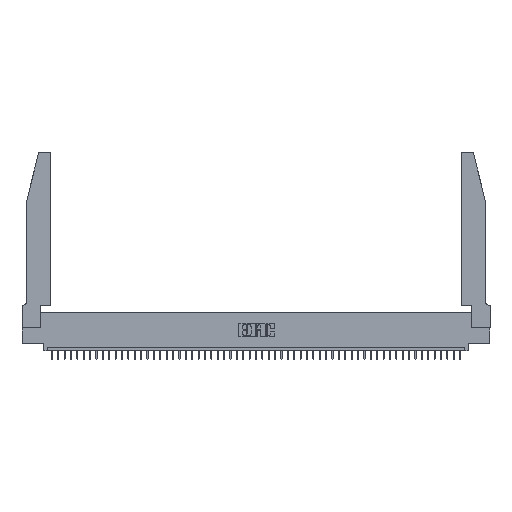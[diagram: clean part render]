
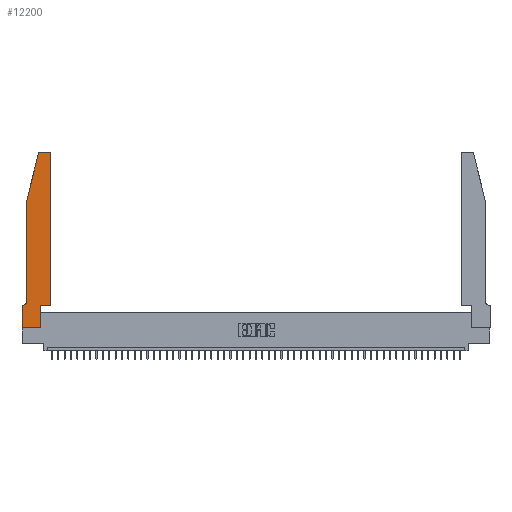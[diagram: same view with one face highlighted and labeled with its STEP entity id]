
A CAD part, top view. The second image highlights one B-rep face of the part: STEP entity #12200.
In plain terms, the highlighted planar face has unit normal (0, 0, 1).
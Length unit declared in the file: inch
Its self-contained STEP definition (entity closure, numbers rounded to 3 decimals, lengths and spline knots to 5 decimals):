
#58 = EDGE_CURVE ( 'NONE', #9470, #3059, #21511, .T. ) ;
#672 = VERTEX_POINT ( 'NONE', #29028 ) ;
#1296 = CARTESIAN_POINT ( 'NONE',  ( 0., 0., 0.37 ) ) ;
#1304 = DIRECTION ( 'NONE',  ( 0., -1., 0. ) ) ;
#2392 = LINE ( 'NONE', #41410, #19967 ) ;
#2555 = EDGE_CURVE ( 'NONE', #45076, #46484, #17953, .T. ) ;
#2768 = AXIS2_PLACEMENT_3D ( 'NONE', #23209, #31160, #35787 ) ;
#2921 = CARTESIAN_POINT ( 'NONE',  ( 0.4505, 2.72, 0.37 ) ) ;
#3059 = VERTEX_POINT ( 'NONE', #1296 ) ;
#3285 = CARTESIAN_POINT ( 'NONE',  ( 0.4205, 2.72, 0.37 ) ) ;
#4116 = EDGE_CURVE ( 'NONE', #12988, #48540, #21064, .T. ) ;
#4312 = DIRECTION ( 'NONE',  ( 0., 0., -1. ) ) ;
#4430 = CARTESIAN_POINT ( 'NONE',  ( 0.0755, 0.35, 0.37 ) ) ;
#5027 = ORIENTED_EDGE ( 'NONE', *, *, #22944, .T. ) ;
#6614 = VECTOR ( 'NONE', #42459, 39.37008 ) ;
#7496 = LINE ( 'NONE', #4430, #47885 ) ;
#7932 = CARTESIAN_POINT ( 'NONE',  ( 0.284, 2.72, 0.37 ) ) ;
#8965 = VERTEX_POINT ( 'NONE', #11845 ) ;
#9470 = VERTEX_POINT ( 'NONE', #25887 ) ;
#9609 = LINE ( 'NONE', #37846, #50065 ) ;
#9868 = ORIENTED_EDGE ( 'NONE', *, *, #12426, .T. ) ;
#9966 = EDGE_CURVE ( 'NONE', #14212, #9470, #7496, .T. ) ;
#10384 = DIRECTION ( 'NONE',  ( 1., 0., 0. ) ) ;
#10969 = DIRECTION ( 'NONE',  ( 0., 0., 1. ) ) ;
#11072 = CIRCLE ( 'NONE', #14379, 0.03 ) ;
#11243 = AXIS2_PLACEMENT_3D ( 'NONE', #20483, #4312, #31771 ) ;
#11390 = PLANE ( 'NONE',  #2768 ) ;
#11602 = DIRECTION ( 'NONE',  ( -1., 0., 0. ) ) ;
#11845 = CARTESIAN_POINT ( 'NONE',  ( 0.284, 2.75, 0.37 ) ) ;
#12200 = ADVANCED_FACE ( 'NONE', ( #46612 ), #11390, .T. ) ;
#12426 = EDGE_CURVE ( 'NONE', #46484, #8965, #2392, .T. ) ;
#12988 = VERTEX_POINT ( 'NONE', #14628 ) ;
#13053 = AXIS2_PLACEMENT_3D ( 'NONE', #3285, #10969, #22793 ) ;
#13166 = ORIENTED_EDGE ( 'NONE', *, *, #58, .T. ) ;
#13350 = DIRECTION ( 'NONE',  ( -0.239, -0.971, 0. ) ) ;
#13462 = ORIENTED_EDGE ( 'NONE', *, *, #22969, .T. ) ;
#13710 = DIRECTION ( 'NONE',  ( 0., 1., 0. ) ) ;
#13948 = VECTOR ( 'NONE', #13710, 39.37008 ) ;
#14212 = VERTEX_POINT ( 'NONE', #38757 ) ;
#14379 = AXIS2_PLACEMENT_3D ( 'NONE', #7932, #32320, #24113 ) ;
#14628 = CARTESIAN_POINT ( 'NONE',  ( 0.0755, 2., 0.37 ) ) ;
#14653 = VERTEX_POINT ( 'NONE', #38193 ) ;
#16464 = VECTOR ( 'NONE', #10384, 39.37008 ) ;
#16563 = EDGE_CURVE ( 'NONE', #48540, #14212, #21930, .T. ) ;
#17202 = CARTESIAN_POINT ( 'NONE',  ( 0.0755, 2., 0.37 ) ) ;
#17310 = CARTESIAN_POINT ( 'NONE',  ( 0.4505, 0.35, 0.37 ) ) ;
#17953 = CIRCLE ( 'NONE', #13053, 0.03 ) ;
#17994 = CARTESIAN_POINT ( 'NONE',  ( 0.4205, 2.75, 0.37 ) ) ;
#19967 = VECTOR ( 'NONE', #41155, 39.37008 ) ;
#20011 = ORIENTED_EDGE ( 'NONE', *, *, #30833, .T. ) ;
#20483 = CARTESIAN_POINT ( 'NONE',  ( 0.0055, 0.42, 0.37 ) ) ;
#21064 = LINE ( 'NONE', #25414, #48483 ) ;
#21511 = LINE ( 'NONE', #37184, #28459 ) ;
#21930 = CIRCLE ( 'NONE', #11243, 0.07 ) ;
#22286 = ORIENTED_EDGE ( 'NONE', *, *, #2555, .T. ) ;
#22441 = LINE ( 'NONE', #33747, #16464 ) ;
#22793 = DIRECTION ( 'NONE',  ( 1., 0., 0. ) ) ;
#22944 = EDGE_CURVE ( 'NONE', #14653, #45076, #36853, .T. ) ;
#22969 = EDGE_CURVE ( 'NONE', #28114, #672, #9609, .T. ) ;
#23209 = CARTESIAN_POINT ( 'NONE',  ( 0., 0.35, 0.37 ) ) ;
#24113 = DIRECTION ( 'NONE',  ( 1., 0., 0. ) ) ;
#24419 = EDGE_CURVE ( 'NONE', #3059, #28114, #27297, .T. ) ;
#24710 = EDGE_LOOP ( 'NONE', ( #9868, #20011, #31247, #25897, #38358, #29701, #13166, #38920, #13462, #40900, #5027, #22286 ) ) ;
#25270 = DIRECTION ( 'NONE',  ( 0., 1., 0. ) ) ;
#25414 = CARTESIAN_POINT ( 'NONE',  ( 0.0755, 2., 0.37 ) ) ;
#25887 = CARTESIAN_POINT ( 'NONE',  ( 0., 0.35, 0.37 ) ) ;
#25897 = ORIENTED_EDGE ( 'NONE', *, *, #4116, .T. ) ;
#26798 = CARTESIAN_POINT ( 'NONE',  ( 0., 0., 0.37 ) ) ;
#27297 = LINE ( 'NONE', #26798, #6614 ) ;
#27520 = EDGE_CURVE ( 'NONE', #47605, #12988, #29017, .T. ) ;
#28114 = VERTEX_POINT ( 'NONE', #45655 ) ;
#28459 = VECTOR ( 'NONE', #48783, 39.37008 ) ;
#29017 = LINE ( 'NONE', #17202, #39713 ) ;
#29028 = CARTESIAN_POINT ( 'NONE',  ( 0.2865, 0.35, 0.37 ) ) ;
#29701 = ORIENTED_EDGE ( 'NONE', *, *, #9966, .T. ) ;
#30833 = EDGE_CURVE ( 'NONE', #8965, #47605, #11072, .T. ) ;
#31160 = DIRECTION ( 'NONE',  ( 0., 0., 1. ) ) ;
#31247 = ORIENTED_EDGE ( 'NONE', *, *, #27520, .T. ) ;
#31771 = DIRECTION ( 'NONE',  ( -1., 0., 0. ) ) ;
#32320 = DIRECTION ( 'NONE',  ( 0., 0., 1. ) ) ;
#33747 = CARTESIAN_POINT ( 'NONE',  ( 0.4505, 0.35, 0.37 ) ) ;
#35787 = DIRECTION ( 'NONE',  ( 1., 0., 0. ) ) ;
#36853 = LINE ( 'NONE', #17310, #13948 ) ;
#37179 = CARTESIAN_POINT ( 'NONE',  ( 0.0755, 0.42, 0.37 ) ) ;
#37184 = CARTESIAN_POINT ( 'NONE',  ( 0., 0., 0.37 ) ) ;
#37846 = CARTESIAN_POINT ( 'NONE',  ( 0.2865, 0.35, 0.37 ) ) ;
#38193 = CARTESIAN_POINT ( 'NONE',  ( 0.4505, 0.35, 0.37 ) ) ;
#38358 = ORIENTED_EDGE ( 'NONE', *, *, #16563, .T. ) ;
#38757 = CARTESIAN_POINT ( 'NONE',  ( 0.0055, 0.35, 0.37 ) ) ;
#38920 = ORIENTED_EDGE ( 'NONE', *, *, #24419, .T. ) ;
#39713 = VECTOR ( 'NONE', #13350, 39.37008 ) ;
#40900 = ORIENTED_EDGE ( 'NONE', *, *, #47330, .T. ) ;
#41155 = DIRECTION ( 'NONE',  ( -1., 0., 0. ) ) ;
#41410 = CARTESIAN_POINT ( 'NONE',  ( 0.2605, 2.75, 0.37 ) ) ;
#42459 = DIRECTION ( 'NONE',  ( 1., 0., 0. ) ) ;
#45076 = VERTEX_POINT ( 'NONE', #2921 ) ;
#45655 = CARTESIAN_POINT ( 'NONE',  ( 0.2865, 0., 0.37 ) ) ;
#46484 = VERTEX_POINT ( 'NONE', #17994 ) ;
#46612 = FACE_OUTER_BOUND ( 'NONE', #24710, .T. ) ;
#47330 = EDGE_CURVE ( 'NONE', #672, #14653, #22441, .T. ) ;
#47605 = VERTEX_POINT ( 'NONE', #48134 ) ;
#47885 = VECTOR ( 'NONE', #11602, 39.37008 ) ;
#48134 = CARTESIAN_POINT ( 'NONE',  ( 0.25487, 2.72718, 0.37 ) ) ;
#48483 = VECTOR ( 'NONE', #1304, 39.37008 ) ;
#48540 = VERTEX_POINT ( 'NONE', #37179 ) ;
#48783 = DIRECTION ( 'NONE',  ( 0., -1., 0. ) ) ;
#50065 = VECTOR ( 'NONE', #25270, 39.37008 ) ;
